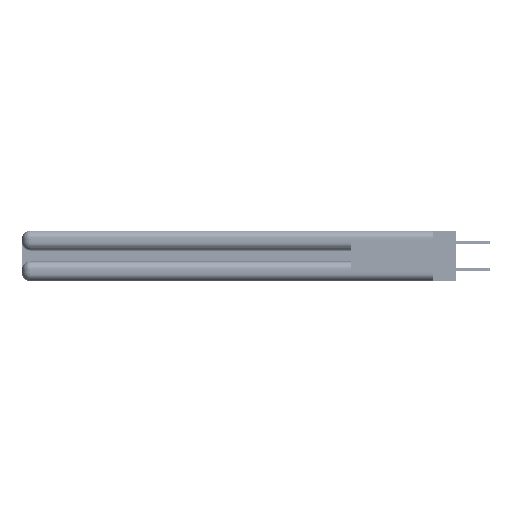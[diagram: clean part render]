
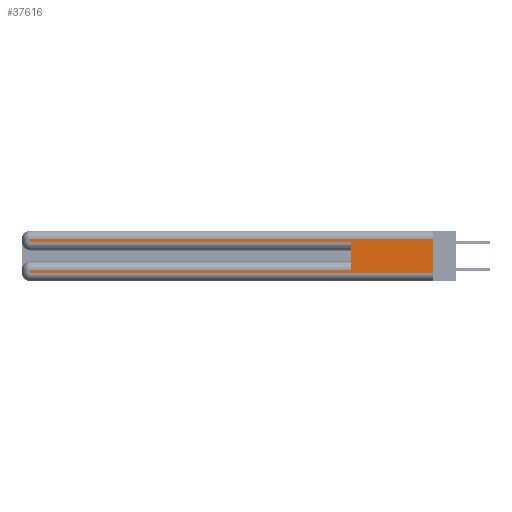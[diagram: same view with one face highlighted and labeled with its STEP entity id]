
A CAD part, left-side view. The second image highlights one B-rep face of the part: STEP entity #37616.
In plain terms, the highlighted planar face has unit normal (-1, 0, 0).
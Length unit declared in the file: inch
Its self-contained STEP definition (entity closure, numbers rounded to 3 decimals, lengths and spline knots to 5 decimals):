
#376 = CARTESIAN_POINT ( 'NONE',  ( 0., 2.94, 0.37 ) ) ;
#837 = VERTEX_POINT ( 'NONE', #9414 ) ;
#875 = CARTESIAN_POINT ( 'NONE',  ( 0., 2.94, 0.285 ) ) ;
#903 = ORIENTED_EDGE ( 'NONE', *, *, #6146, .T. ) ;
#2736 = ORIENTED_EDGE ( 'NONE', *, *, #44527, .T. ) ;
#3005 = CARTESIAN_POINT ( 'NONE',  ( 0., 0., 0.31 ) ) ;
#4772 = DIRECTION ( 'NONE',  ( 1., 0., 0. ) ) ;
#5404 = LINE ( 'NONE', #36178, #5972 ) ;
#5972 = VECTOR ( 'NONE', #43923, 39.37008 ) ;
#6009 = VECTOR ( 'NONE', #25867, 39.37008 ) ;
#6146 = EDGE_CURVE ( 'NONE', #35634, #22382, #12097, .T. ) ;
#7003 = CARTESIAN_POINT ( 'NONE',  ( 0., 0., 0.085 ) ) ;
#7370 = CARTESIAN_POINT ( 'NONE',  ( 0., 0., 0.37 ) ) ;
#9355 = VERTEX_POINT ( 'NONE', #33862 ) ;
#9414 = CARTESIAN_POINT ( 'NONE',  ( 0., 0.6, 0.085 ) ) ;
#10704 = ORIENTED_EDGE ( 'NONE', *, *, #14305, .T. ) ;
#12097 = LINE ( 'NONE', #3005, #15729 ) ;
#12686 = CARTESIAN_POINT ( 'NONE',  ( 0., 0.6, 0.145 ) ) ;
#14305 = EDGE_CURVE ( 'NONE', #40814, #18174, #32578, .T. ) ;
#14502 = DIRECTION ( 'NONE',  ( 0., 1., 0. ) ) ;
#15729 = VECTOR ( 'NONE', #33460, 39.37008 ) ;
#16049 = EDGE_CURVE ( 'NONE', #9355, #33619, #5404, .T. ) ;
#16534 = CARTESIAN_POINT ( 'NONE',  ( 0., 0., 0.285 ) ) ;
#18174 = VERTEX_POINT ( 'NONE', #23826 ) ;
#18850 = CARTESIAN_POINT ( 'NONE',  ( 0., 2.94, 0.06 ) ) ;
#19969 = VECTOR ( 'NONE', #47603, 39.37008 ) ;
#20715 = CARTESIAN_POINT ( 'NONE',  ( 0., 0., 0.06 ) ) ;
#21821 = LINE ( 'NONE', #12686, #43191 ) ;
#22382 = VERTEX_POINT ( 'NONE', #28774 ) ;
#22935 = CARTESIAN_POINT ( 'NONE',  ( 0., 0., 0.31 ) ) ;
#23039 = ORIENTED_EDGE ( 'NONE', *, *, #16049, .T. ) ;
#23647 = AXIS2_PLACEMENT_3D ( 'NONE', #42815, #4772, #39009 ) ;
#23826 = CARTESIAN_POINT ( 'NONE',  ( 0., 0.6, 0.285 ) ) ;
#23831 = VECTOR ( 'NONE', #30560, 39.37008 ) ;
#25867 = DIRECTION ( 'NONE',  ( 0., 0., -1. ) ) ;
#26280 = EDGE_CURVE ( 'NONE', #837, #18174, #21821, .T. ) ;
#26656 = LINE ( 'NONE', #7003, #27847 ) ;
#26716 = ORIENTED_EDGE ( 'NONE', *, *, #26280, .F. ) ;
#27847 = VECTOR ( 'NONE', #14502, 39.37008 ) ;
#28774 = CARTESIAN_POINT ( 'NONE',  ( 0., 2.94, 0.31 ) ) ;
#30560 = DIRECTION ( 'NONE',  ( 0., 0., -1. ) ) ;
#31683 = VERTEX_POINT ( 'NONE', #43529 ) ;
#32578 = LINE ( 'NONE', #16534, #48615 ) ;
#33103 = EDGE_CURVE ( 'NONE', #22382, #40814, #48783, .T. ) ;
#33460 = DIRECTION ( 'NONE',  ( 0., 1., 0. ) ) ;
#33530 = ORIENTED_EDGE ( 'NONE', *, *, #42388, .T. ) ;
#33619 = VERTEX_POINT ( 'NONE', #18850 ) ;
#33862 = CARTESIAN_POINT ( 'NONE',  ( 0., 2.94, 0.085 ) ) ;
#35233 = PLANE ( 'NONE',  #23647 ) ;
#35634 = VERTEX_POINT ( 'NONE', #22935 ) ;
#35790 = LINE ( 'NONE', #7370, #6009 ) ;
#36178 = CARTESIAN_POINT ( 'NONE',  ( 0., 2.94, 0.37 ) ) ;
#36506 = FACE_OUTER_BOUND ( 'NONE', #48775, .T. ) ;
#37616 = ADVANCED_FACE ( 'NONE', ( #36506 ), #35233, .F. ) ;
#39009 = DIRECTION ( 'NONE',  ( 0., 0., -1. ) ) ;
#39258 = DIRECTION ( 'NONE',  ( 0., 0., 1. ) ) ;
#40144 = LINE ( 'NONE', #20715, #19969 ) ;
#40814 = VERTEX_POINT ( 'NONE', #875 ) ;
#41937 = ORIENTED_EDGE ( 'NONE', *, *, #48708, .F. ) ;
#42388 = EDGE_CURVE ( 'NONE', #837, #9355, #26656, .T. ) ;
#42815 = CARTESIAN_POINT ( 'NONE',  ( 0., 0., 0.37 ) ) ;
#43191 = VECTOR ( 'NONE', #39258, 39.37008 ) ;
#43529 = CARTESIAN_POINT ( 'NONE',  ( 0., 0., 0.06 ) ) ;
#43579 = ORIENTED_EDGE ( 'NONE', *, *, #33103, .T. ) ;
#43923 = DIRECTION ( 'NONE',  ( 0., 0., -1. ) ) ;
#44527 = EDGE_CURVE ( 'NONE', #33619, #31683, #40144, .T. ) ;
#47412 = DIRECTION ( 'NONE',  ( 0., -1., 0. ) ) ;
#47603 = DIRECTION ( 'NONE',  ( 0., -1., 0. ) ) ;
#48615 = VECTOR ( 'NONE', #47412, 39.37008 ) ;
#48708 = EDGE_CURVE ( 'NONE', #35634, #31683, #35790, .T. ) ;
#48775 = EDGE_LOOP ( 'NONE', ( #41937, #903, #43579, #10704, #26716, #33530, #23039, #2736 ) ) ;
#48783 = LINE ( 'NONE', #376, #23831 ) ;
